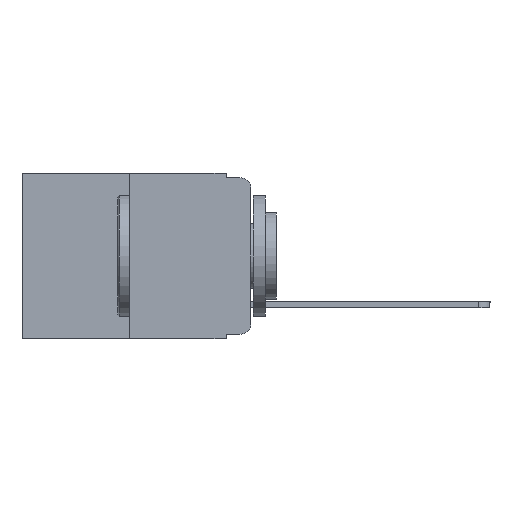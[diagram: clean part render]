
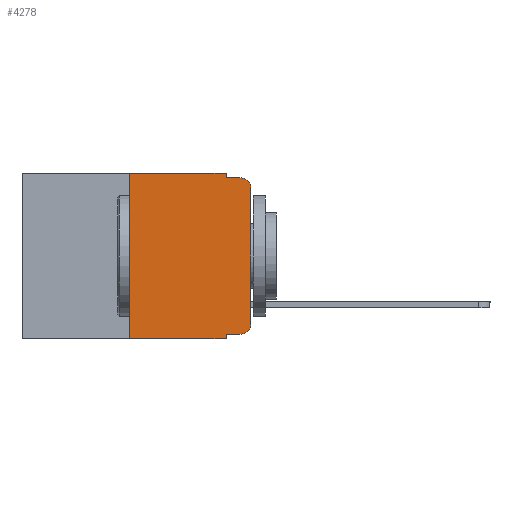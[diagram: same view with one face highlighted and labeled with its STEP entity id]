
A CAD part, left-side view. The second image highlights one B-rep face of the part: STEP entity #4278.
In plain terms, the highlighted planar face has unit normal (-1, 0, 0).
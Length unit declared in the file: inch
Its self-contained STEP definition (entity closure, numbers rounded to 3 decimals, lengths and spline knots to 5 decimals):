
#284 = CARTESIAN_POINT ( 'NONE',  ( 0., 0.02, -0.313 ) ) ;
#313 = ORIENTED_EDGE ( 'NONE', *, *, #5278, .T. ) ;
#669 = ORIENTED_EDGE ( 'NONE', *, *, #13249, .F. ) ;
#1678 = ORIENTED_EDGE ( 'NONE', *, *, #9581, .F. ) ;
#1988 = DIRECTION ( 'NONE',  ( 0., 0., 1. ) ) ;
#2326 = ORIENTED_EDGE ( 'NONE', *, *, #7588, .T. ) ;
#2406 = CARTESIAN_POINT ( 'NONE',  ( 0., 0.051, -0.333 ) ) ;
#2447 = CARTESIAN_POINT ( 'NONE',  ( 0., 0.051, -0.343 ) ) ;
#2600 = CARTESIAN_POINT ( 'NONE',  ( 0., 0.25, 0. ) ) ;
#2899 = EDGE_CURVE ( 'NONE', #2996, #3026, #13142, .T. ) ;
#2996 = VERTEX_POINT ( 'NONE', #12210 ) ;
#3026 = VERTEX_POINT ( 'NONE', #11715 ) ;
#3170 = DIRECTION ( 'NONE',  ( 0., -1., 0. ) ) ;
#3593 = DIRECTION ( 'NONE',  ( 0., -1., 0. ) ) ;
#3948 = VERTEX_POINT ( 'NONE', #2406 ) ;
#4278 = ADVANCED_FACE ( 'NONE', ( #13461 ), #5644, .F. ) ;
#4480 = CARTESIAN_POINT ( 'NONE',  ( 0., 0.051, -0.333 ) ) ;
#4498 = LINE ( 'NONE', #12527, #12128 ) ;
#4961 = EDGE_CURVE ( 'NONE', #3026, #10049, #9592, .T. ) ;
#5278 = EDGE_CURVE ( 'NONE', #8473, #6741, #14186, .T. ) ;
#5279 = EDGE_CURVE ( 'NONE', #8473, #11885, #9616, .T. ) ;
#5442 = DIRECTION ( 'NONE',  ( 0., -1., 0. ) ) ;
#5498 = DIRECTION ( 'NONE',  ( 0., 0., 1. ) ) ;
#5644 = PLANE ( 'NONE',  #12941 ) ;
#5786 = ORIENTED_EDGE ( 'NONE', *, *, #10478, .F. ) ;
#5793 = DIRECTION ( 'NONE',  ( -1., 0., 0. ) ) ;
#5799 = CARTESIAN_POINT ( 'NONE',  ( 0., 0.051, -0.01 ) ) ;
#5897 = DIRECTION ( 'NONE',  ( 0., 0., -1. ) ) ;
#5909 = DIRECTION ( 'NONE',  ( 0., 0., -1. ) ) ;
#6028 = ORIENTED_EDGE ( 'NONE', *, *, #5279, .F. ) ;
#6109 = VECTOR ( 'NONE', #5909, 39.37008 ) ;
#6121 = EDGE_CURVE ( 'NONE', #3948, #2996, #7839, .T. ) ;
#6211 = CARTESIAN_POINT ( 'NONE',  ( 0., 0.25, -0.343 ) ) ;
#6290 = EDGE_LOOP ( 'NONE', ( #12721, #2326, #5786, #1678, #669, #6028, #313, #9647, #14078, #12464 ) ) ;
#6467 = CARTESIAN_POINT ( 'NONE',  ( 0., 0.051, -0.01 ) ) ;
#6740 = DIRECTION ( 'NONE',  ( 0., 0., -1. ) ) ;
#6741 = VERTEX_POINT ( 'NONE', #2447 ) ;
#7588 = EDGE_CURVE ( 'NONE', #10049, #13421, #10014, .T. ) ;
#7605 = CARTESIAN_POINT ( 'NONE',  ( 0., 0.25, 0. ) ) ;
#7839 = LINE ( 'NONE', #4480, #8145 ) ;
#8023 = LINE ( 'NONE', #11383, #6109 ) ;
#8081 = CARTESIAN_POINT ( 'NONE',  ( 0., 0.02, -0.03 ) ) ;
#8145 = VECTOR ( 'NONE', #5442, 39.37008 ) ;
#8473 = VERTEX_POINT ( 'NONE', #6211 ) ;
#8758 = CARTESIAN_POINT ( 'NONE',  ( 0., 0.473, -0.343 ) ) ;
#8997 = DIRECTION ( 'NONE',  ( 0., 0., -1. ) ) ;
#9192 = CARTESIAN_POINT ( 'NONE',  ( 0., 0.02, -0.01 ) ) ;
#9581 = EDGE_CURVE ( 'NONE', #10523, #10208, #8023, .T. ) ;
#9592 = LINE ( 'NONE', #10961, #10419 ) ;
#9616 = LINE ( 'NONE', #7605, #12727 ) ;
#9647 = ORIENTED_EDGE ( 'NONE', *, *, #11286, .F. ) ;
#9865 = VECTOR ( 'NONE', #3593, 39.37008 ) ;
#10014 = CIRCLE ( 'NONE', #10247, 0.02 ) ;
#10049 = VERTEX_POINT ( 'NONE', #13842 ) ;
#10208 = VERTEX_POINT ( 'NONE', #6467 ) ;
#10247 = AXIS2_PLACEMENT_3D ( 'NONE', #8081, #13700, #5897 ) ;
#10294 = CARTESIAN_POINT ( 'NONE',  ( 0., 0.051, 0. ) ) ;
#10419 = VECTOR ( 'NONE', #1988, 39.37008 ) ;
#10478 = EDGE_CURVE ( 'NONE', #10208, #13421, #11280, .T. ) ;
#10523 = VERTEX_POINT ( 'NONE', #10294 ) ;
#10961 = CARTESIAN_POINT ( 'NONE',  ( 0., 0., 0. ) ) ;
#11195 = LINE ( 'NONE', #13523, #9865 ) ;
#11280 = LINE ( 'NONE', #5799, #11425 ) ;
#11286 = EDGE_CURVE ( 'NONE', #3948, #6741, #4498, .T. ) ;
#11383 = CARTESIAN_POINT ( 'NONE',  ( 0., 0.051, 0. ) ) ;
#11425 = VECTOR ( 'NONE', #13251, 39.37008 ) ;
#11560 = VECTOR ( 'NONE', #3170, 39.37008 ) ;
#11715 = CARTESIAN_POINT ( 'NONE',  ( 0., 0., -0.313 ) ) ;
#11885 = VERTEX_POINT ( 'NONE', #2600 ) ;
#12128 = VECTOR ( 'NONE', #8997, 39.37008 ) ;
#12192 = AXIS2_PLACEMENT_3D ( 'NONE', #284, #5793, #6740 ) ;
#12210 = CARTESIAN_POINT ( 'NONE',  ( 0., 0.02, -0.333 ) ) ;
#12283 = DIRECTION ( 'NONE',  ( 1., 0., 0. ) ) ;
#12357 = CARTESIAN_POINT ( 'NONE',  ( 0., 0.473, 0. ) ) ;
#12464 = ORIENTED_EDGE ( 'NONE', *, *, #2899, .T. ) ;
#12527 = CARTESIAN_POINT ( 'NONE',  ( 0., 0.051, 0. ) ) ;
#12721 = ORIENTED_EDGE ( 'NONE', *, *, #4961, .T. ) ;
#12727 = VECTOR ( 'NONE', #5498, 39.37008 ) ;
#12941 = AXIS2_PLACEMENT_3D ( 'NONE', #12357, #12283, #13676 ) ;
#13142 = CIRCLE ( 'NONE', #12192, 0.02 ) ;
#13249 = EDGE_CURVE ( 'NONE', #11885, #10523, #11195, .T. ) ;
#13251 = DIRECTION ( 'NONE',  ( 0., -1., 0. ) ) ;
#13421 = VERTEX_POINT ( 'NONE', #9192 ) ;
#13461 = FACE_OUTER_BOUND ( 'NONE', #6290, .T. ) ;
#13523 = CARTESIAN_POINT ( 'NONE',  ( 0., 0.473, 0. ) ) ;
#13676 = DIRECTION ( 'NONE',  ( 0., 0., -1. ) ) ;
#13700 = DIRECTION ( 'NONE',  ( -1., 0., 0. ) ) ;
#13842 = CARTESIAN_POINT ( 'NONE',  ( 0., 0., -0.03 ) ) ;
#14078 = ORIENTED_EDGE ( 'NONE', *, *, #6121, .T. ) ;
#14186 = LINE ( 'NONE', #8758, #11560 ) ;
